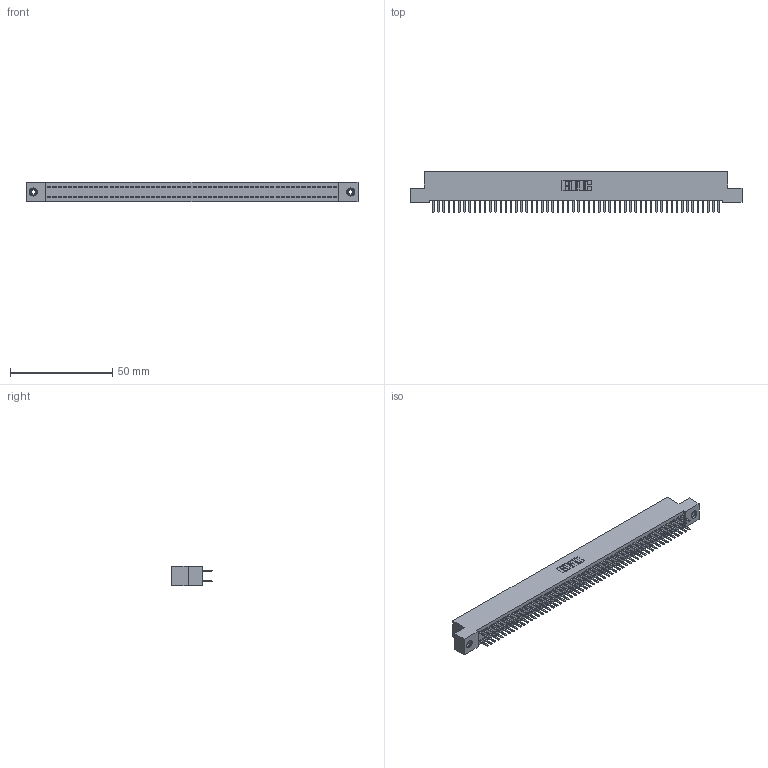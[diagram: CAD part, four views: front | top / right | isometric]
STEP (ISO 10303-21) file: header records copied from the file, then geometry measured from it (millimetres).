
FILE_DESCRIPTION (( 'STEP AP203' ), '1' );
FILE_NAME ('392-112-520-208.STEP', '2018-08-18T22:14:42', ( '' ), ( '' ), 'SwSTEP 2.0', 'SolidWorks 2016', '' );
FILE_SCHEMA (( 'CONFIG_CONTROL_DESIGN' ));
Length unit declared in the file: inch
Products named in the file (4): 342 Part_TI; 345-292-001_345-293-120; 345-250-001_345-250-003-102; 392-112-520-208
Assembly tree (115 placements, depth 2):
  392-112-520-208
    342 Part_TI
    345-292-001_345-293-120  x112
    345-250-001_345-250-003-102  x2
Bounding box: 162.56 x 20.02 x 9.4 mm (x, y, z)
Volume: 14617.3 mm3; surface area: 24032.5 mm2
Topology: 115 solids, 115 shells, 6442 faces, 18691 edges, 12154 vertices
Faces by surface type: plane 4354, cylinder 2072, cone 12, torus 4
Entity records: 35384 total; most frequent: CARTESIAN_POINT 5841, ORIENTED_EDGE 5758, DIRECTION 4985, EDGE_CURVE 2879, VECTOR 2727, LINE 2727, VERTEX_POINT 1912, AXIS2_PLACEMENT_3D 1129
